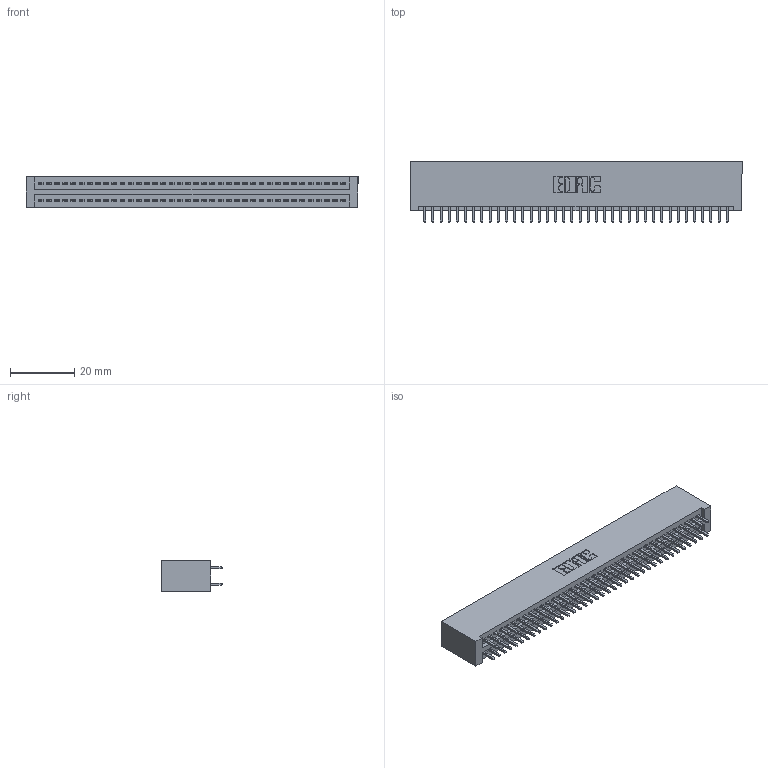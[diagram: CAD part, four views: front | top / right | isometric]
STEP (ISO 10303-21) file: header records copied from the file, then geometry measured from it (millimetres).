
FILE_DESCRIPTION (( 'STEP AP203' ), '1' );
FILE_NAME ('395-076-521-201.STEP', '2018-11-27T20:35:37', ( '' ), ( '' ), 'SwSTEP 2.0', 'SolidWorks 2016', '' );
FILE_SCHEMA (( 'CONFIG_CONTROL_DESIGN' ));
Length unit declared in the file: inch
Products named in the file (3): 345 Part_No Mounting Lugs; 395-076-521-201; 345-292-001_345-293-121
Assembly tree (77 placements, depth 2):
  395-076-521-201
    345 Part_No Mounting Lugs
    345-292-001_345-293-121  x76
Bounding box: 103.12 x 18.72 x 9.4 mm (x, y, z)
Volume: 10565.3 mm3; surface area: 15641.2 mm2
Topology: 77 solids, 77 shells, 3918 faces, 11641 edges, 7658 vertices
Faces by surface type: plane 2584, cylinder 1334
Entity records: 30095 total; most frequent: CARTESIAN_POINT 5048, ORIENTED_EDGE 4982, DIRECTION 4451, EDGE_CURVE 2491, LINE 2215, VECTOR 2215, VERTEX_POINT 1658, AXIS2_PLACEMENT_3D 1118
